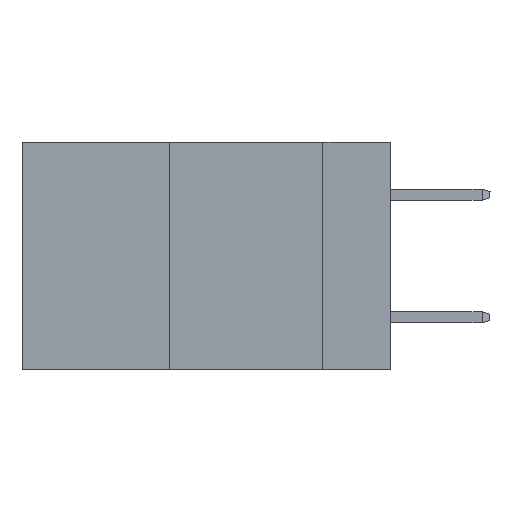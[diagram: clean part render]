
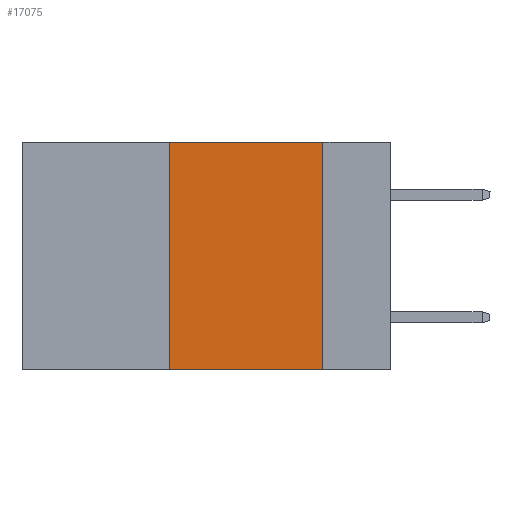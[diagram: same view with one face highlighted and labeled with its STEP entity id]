
A CAD part, left-side view. The second image highlights one B-rep face of the part: STEP entity #17075.
In plain terms, the highlighted planar face has unit normal (-1, 0, 0).
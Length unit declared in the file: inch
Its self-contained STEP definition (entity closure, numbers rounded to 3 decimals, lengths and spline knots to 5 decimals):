
#496 = DIRECTION ( 'NONE',  ( 0., 0., 1. ) ) ;
#530 = AXIS2_PLACEMENT_3D ( 'NONE', #12944, #17728, #15202 ) ;
#1153 = VERTEX_POINT ( 'NONE', #3877 ) ;
#1221 = PLANE ( 'NONE',  #530 ) ;
#1443 = ORIENTED_EDGE ( 'NONE', *, *, #20962, .F. ) ;
#1631 = DIRECTION ( 'NONE',  ( 0., -1., 0. ) ) ;
#3259 = VECTOR ( 'NONE', #5806, 39.37008 ) ;
#3720 = DIRECTION ( 'NONE',  ( 0., -1., 0. ) ) ;
#3877 = CARTESIAN_POINT ( 'NONE',  ( 0., 0.36, -0.37 ) ) ;
#5316 = LINE ( 'NONE', #12239, #6909 ) ;
#5580 = EDGE_CURVE ( 'NONE', #25844, #15505, #15276, .T. ) ;
#5806 = DIRECTION ( 'NONE',  ( 0., 0., -1. ) ) ;
#6724 = VECTOR ( 'NONE', #3720, 39.37008 ) ;
#6909 = VECTOR ( 'NONE', #496, 39.37008 ) ;
#8243 = LINE ( 'NONE', #17401, #20781 ) ;
#8382 = LINE ( 'NONE', #28976, #6724 ) ;
#8722 = EDGE_LOOP ( 'NONE', ( #22298, #1443, #9579, #14144 ) ) ;
#9579 = ORIENTED_EDGE ( 'NONE', *, *, #15110, .F. ) ;
#10612 = CARTESIAN_POINT ( 'NONE',  ( 0., 0.11, 0. ) ) ;
#11307 = CARTESIAN_POINT ( 'NONE',  ( 0., 0.11, -0.37 ) ) ;
#12239 = CARTESIAN_POINT ( 'NONE',  ( 0., 0.36, 0. ) ) ;
#12944 = CARTESIAN_POINT ( 'NONE',  ( 0., 0.6, 0. ) ) ;
#14144 = ORIENTED_EDGE ( 'NONE', *, *, #17839, .T. ) ;
#15110 = EDGE_CURVE ( 'NONE', #1153, #29698, #5316, .T. ) ;
#15202 = DIRECTION ( 'NONE',  ( 0., 0., -1. ) ) ;
#15276 = LINE ( 'NONE', #10612, #3259 ) ;
#15505 = VERTEX_POINT ( 'NONE', #11307 ) ;
#17075 = ADVANCED_FACE ( 'NONE', ( #19405 ), #1221, .F. ) ;
#17401 = CARTESIAN_POINT ( 'NONE',  ( 0., 0.6, 0. ) ) ;
#17728 = DIRECTION ( 'NONE',  ( 1., 0., 0. ) ) ;
#17839 = EDGE_CURVE ( 'NONE', #1153, #15505, #8382, .T. ) ;
#18498 = CARTESIAN_POINT ( 'NONE',  ( 0., 0.36, 0. ) ) ;
#19405 = FACE_OUTER_BOUND ( 'NONE', #8722, .T. ) ;
#20781 = VECTOR ( 'NONE', #1631, 39.37008 ) ;
#20962 = EDGE_CURVE ( 'NONE', #29698, #25844, #8243, .T. ) ;
#22298 = ORIENTED_EDGE ( 'NONE', *, *, #5580, .F. ) ;
#24427 = CARTESIAN_POINT ( 'NONE',  ( 0., 0.11, 0. ) ) ;
#25844 = VERTEX_POINT ( 'NONE', #24427 ) ;
#28976 = CARTESIAN_POINT ( 'NONE',  ( 0., 0.6, -0.37 ) ) ;
#29698 = VERTEX_POINT ( 'NONE', #18498 ) ;
